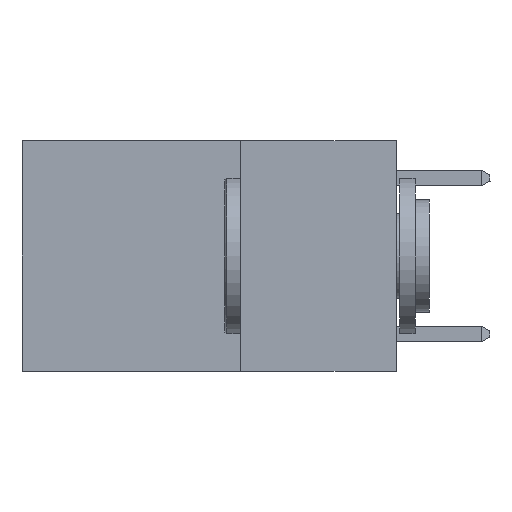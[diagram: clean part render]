
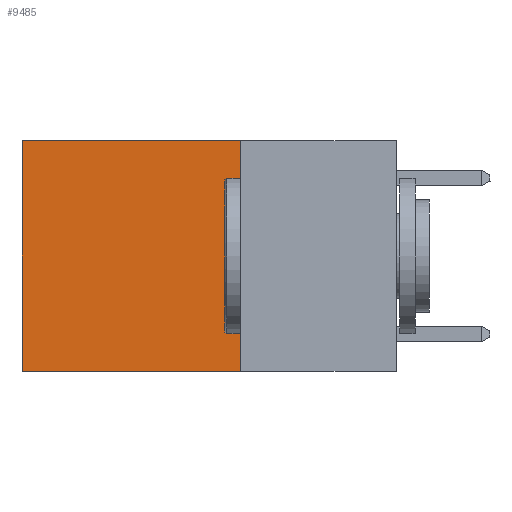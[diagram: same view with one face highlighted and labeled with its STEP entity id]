
A CAD part, left-side view. The second image highlights one B-rep face of the part: STEP entity #9485.
In plain terms, the highlighted planar face has unit normal (-1, 0, 0).
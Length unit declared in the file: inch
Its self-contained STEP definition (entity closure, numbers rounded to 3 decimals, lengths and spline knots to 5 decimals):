
#667 = EDGE_CURVE ( 'NONE', #2364, #3654, #1861, .T. ) ;
#1530 = CARTESIAN_POINT ( 'NONE',  ( 0.2625, 0.25, 0. ) ) ;
#1861 = LINE ( 'NONE', #18325, #6624 ) ;
#2364 = VERTEX_POINT ( 'NONE', #16331 ) ;
#2721 = CARTESIAN_POINT ( 'NONE',  ( 0.2625, 0.25, -0.37 ) ) ;
#3281 = PLANE ( 'NONE',  #18023 ) ;
#3293 = DIRECTION ( 'NONE',  ( 0., 0., -1. ) ) ;
#3314 = EDGE_CURVE ( 'NONE', #9971, #3654, #11554, .T. ) ;
#3654 = VERTEX_POINT ( 'NONE', #16277 ) ;
#5673 = EDGE_CURVE ( 'NONE', #9180, #2364, #12281, .T. ) ;
#6624 = VECTOR ( 'NONE', #3293, 39.37008 ) ;
#7460 = DIRECTION ( 'NONE',  ( 1., 0., 0. ) ) ;
#8578 = VECTOR ( 'NONE', #19915, 39.37008 ) ;
#8762 = DIRECTION ( 'NONE',  ( 0., 1., 0. ) ) ;
#9180 = VERTEX_POINT ( 'NONE', #19298 ) ;
#9485 = ADVANCED_FACE ( 'NONE', ( #13550 ), #3281, .F. ) ;
#9971 = VERTEX_POINT ( 'NONE', #10622 ) ;
#10622 = CARTESIAN_POINT ( 'NONE',  ( 0.2625, 0.25, -0.37 ) ) ;
#11554 = LINE ( 'NONE', #2721, #8578 ) ;
#12281 = LINE ( 'NONE', #1530, #13453 ) ;
#12954 = CARTESIAN_POINT ( 'NONE',  ( 0.2625, 0.25, 0. ) ) ;
#12991 = ORIENTED_EDGE ( 'NONE', *, *, #667, .T. ) ;
#13453 = VECTOR ( 'NONE', #8762, 39.37008 ) ;
#13550 = FACE_OUTER_BOUND ( 'NONE', #13682, .T. ) ;
#13682 = EDGE_LOOP ( 'NONE', ( #12991, #15376, #22680, #14054 ) ) ;
#14054 = ORIENTED_EDGE ( 'NONE', *, *, #5673, .T. ) ;
#14779 = VECTOR ( 'NONE', #20359, 39.37008 ) ;
#14991 = DIRECTION ( 'NONE',  ( 0., 0., -1. ) ) ;
#15376 = ORIENTED_EDGE ( 'NONE', *, *, #3314, .F. ) ;
#15863 = EDGE_CURVE ( 'NONE', #9180, #9971, #23965, .T. ) ;
#16277 = CARTESIAN_POINT ( 'NONE',  ( 0.2625, 0.6, -0.37 ) ) ;
#16331 = CARTESIAN_POINT ( 'NONE',  ( 0.2625, 0.6, 0. ) ) ;
#18023 = AXIS2_PLACEMENT_3D ( 'NONE', #12954, #7460, #14991 ) ;
#18325 = CARTESIAN_POINT ( 'NONE',  ( 0.2625, 0.6, 0. ) ) ;
#19298 = CARTESIAN_POINT ( 'NONE',  ( 0.2625, 0.25, 0. ) ) ;
#19915 = DIRECTION ( 'NONE',  ( 0., 1., 0. ) ) ;
#20359 = DIRECTION ( 'NONE',  ( 0., 0., -1. ) ) ;
#22464 = CARTESIAN_POINT ( 'NONE',  ( 0.2625, 0.25, 0. ) ) ;
#22680 = ORIENTED_EDGE ( 'NONE', *, *, #15863, .F. ) ;
#23965 = LINE ( 'NONE', #22464, #14779 ) ;
